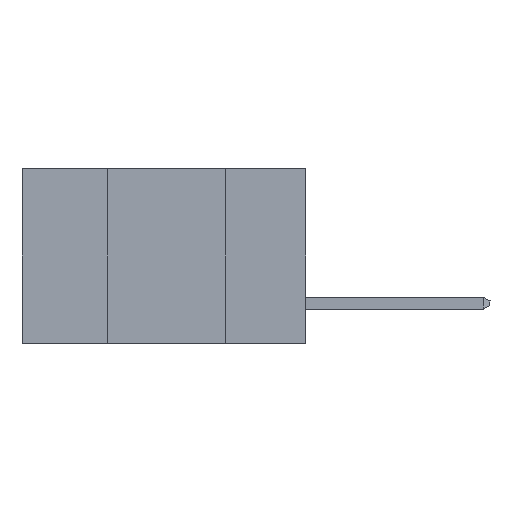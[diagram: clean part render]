
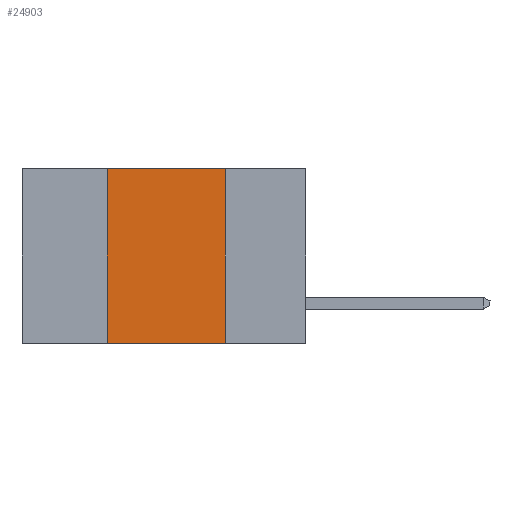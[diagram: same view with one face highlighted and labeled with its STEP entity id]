
A CAD part, left-side view. The second image highlights one B-rep face of the part: STEP entity #24903.
In plain terms, the highlighted planar face has unit normal (-1, 0, 0).
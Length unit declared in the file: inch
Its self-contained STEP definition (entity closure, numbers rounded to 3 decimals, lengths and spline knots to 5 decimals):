
#11 = LINE ( 'NONE', #4065, #4402 ) ;
#455 = EDGE_CURVE ( 'NONE', #4541, #24455, #12372, .T. ) ;
#789 = CARTESIAN_POINT ( 'NONE',  ( 0., 0.17, -0.37 ) ) ;
#1908 = CARTESIAN_POINT ( 'NONE',  ( 0., 0.17, 0. ) ) ;
#2253 = DIRECTION ( 'NONE',  ( 0., -1., 0. ) ) ;
#3111 = LINE ( 'NONE', #7653, #20916 ) ;
#3591 = ORIENTED_EDGE ( 'NONE', *, *, #27327, .F. ) ;
#4065 = CARTESIAN_POINT ( 'NONE',  ( 0., 0.6, -0.37 ) ) ;
#4249 = DIRECTION ( 'NONE',  ( 0., 0., -1. ) ) ;
#4402 = VECTOR ( 'NONE', #6404, 39.37008 ) ;
#4541 = VERTEX_POINT ( 'NONE', #15791 ) ;
#5057 = ORIENTED_EDGE ( 'NONE', *, *, #24022, .T. ) ;
#5989 = AXIS2_PLACEMENT_3D ( 'NONE', #23131, #20807, #9710 ) ;
#6211 = EDGE_CURVE ( 'NONE', #24455, #20340, #25261, .T. ) ;
#6359 = ORIENTED_EDGE ( 'NONE', *, *, #6211, .F. ) ;
#6404 = DIRECTION ( 'NONE',  ( 0., -1., 0. ) ) ;
#7653 = CARTESIAN_POINT ( 'NONE',  ( 0., 0.42, 0. ) ) ;
#9710 = DIRECTION ( 'NONE',  ( 0., 0., -1. ) ) ;
#11170 = CARTESIAN_POINT ( 'NONE',  ( 0., 0.6, 0. ) ) ;
#12018 = VERTEX_POINT ( 'NONE', #28092 ) ;
#12372 = LINE ( 'NONE', #11170, #18568 ) ;
#15791 = CARTESIAN_POINT ( 'NONE',  ( 0., 0.42, 0. ) ) ;
#16478 = PLANE ( 'NONE',  #5989 ) ;
#18052 = ORIENTED_EDGE ( 'NONE', *, *, #455, .F. ) ;
#18568 = VECTOR ( 'NONE', #2253, 39.37008 ) ;
#20340 = VERTEX_POINT ( 'NONE', #789 ) ;
#20807 = DIRECTION ( 'NONE',  ( 1., 0., 0. ) ) ;
#20916 = VECTOR ( 'NONE', #28851, 39.37008 ) ;
#21455 = FACE_OUTER_BOUND ( 'NONE', #25874, .T. ) ;
#23131 = CARTESIAN_POINT ( 'NONE',  ( 0., 0.6, 0. ) ) ;
#23844 = VECTOR ( 'NONE', #4249, 39.37008 ) ;
#24022 = EDGE_CURVE ( 'NONE', #12018, #20340, #11, .T. ) ;
#24455 = VERTEX_POINT ( 'NONE', #26380 ) ;
#24903 = ADVANCED_FACE ( 'NONE', ( #21455 ), #16478, .F. ) ;
#25261 = LINE ( 'NONE', #1908, #23844 ) ;
#25874 = EDGE_LOOP ( 'NONE', ( #6359, #18052, #3591, #5057 ) ) ;
#26380 = CARTESIAN_POINT ( 'NONE',  ( 0., 0.17, 0. ) ) ;
#27327 = EDGE_CURVE ( 'NONE', #12018, #4541, #3111, .T. ) ;
#28092 = CARTESIAN_POINT ( 'NONE',  ( 0., 0.42, -0.37 ) ) ;
#28851 = DIRECTION ( 'NONE',  ( 0., 0., 1. ) ) ;
